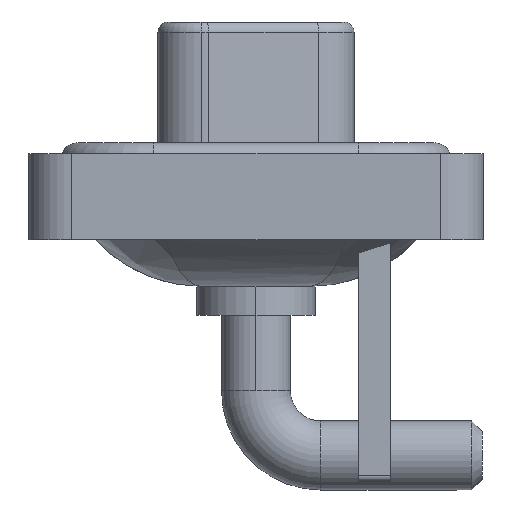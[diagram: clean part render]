
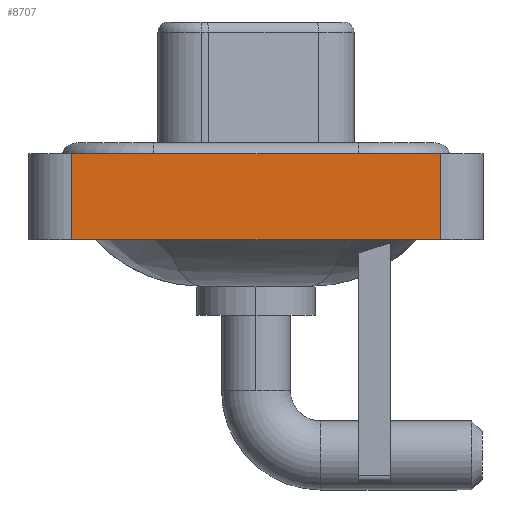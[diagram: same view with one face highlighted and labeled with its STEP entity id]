
A CAD part, left-side view. The second image highlights one B-rep face of the part: STEP entity #8707.
In plain terms, the highlighted planar face has unit normal (-1, 0, 0).
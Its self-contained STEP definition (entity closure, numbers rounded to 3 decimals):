
#892 = ORIENTED_EDGE ( 'NONE', *, *, #13719, .F. ) ;
#903 = DIRECTION ( 'NONE',  ( 0., 0., 1. ) ) ;
#2078 = LINE ( 'NONE', #10963, #12333 ) ;
#3407 = CARTESIAN_POINT ( 'NONE',  ( -7.25, 8.55, -3.6 ) ) ;
#3784 = ORIENTED_EDGE ( 'NONE', *, *, #5204, .T. ) ;
#4314 = DIRECTION ( 'NONE',  ( 0., 0., 1. ) ) ;
#5204 = EDGE_CURVE ( 'NONE', #14018, #8921, #15393, .T. ) ;
#5382 = AXIS2_PLACEMENT_3D ( 'NONE', #10099, #7242, #4314 ) ;
#5666 = VERTEX_POINT ( 'NONE', #15191 ) ;
#6091 = ORIENTED_EDGE ( 'NONE', *, *, #15179, .T. ) ;
#6730 = LINE ( 'NONE', #12501, #16020 ) ;
#6797 = DIRECTION ( 'NONE',  ( 0., -1., 0. ) ) ;
#7242 = DIRECTION ( 'NONE',  ( -1., 0., 0. ) ) ;
#7818 = DIRECTION ( 'NONE',  ( 0., -1., 0. ) ) ;
#8166 = CARTESIAN_POINT ( 'NONE',  ( -7.25, -8.55, -3.6 ) ) ;
#8707 = ADVANCED_FACE ( 'NONE', ( #10189 ), #17540, .T. ) ;
#8921 = VERTEX_POINT ( 'NONE', #8166 ) ;
#8945 = CARTESIAN_POINT ( 'NONE',  ( -7.25, 8.55, 0.4 ) ) ;
#9672 = LINE ( 'NONE', #18436, #15442 ) ;
#10099 = CARTESIAN_POINT ( 'NONE',  ( -7.25, -8.55, -3.6 ) ) ;
#10189 = FACE_OUTER_BOUND ( 'NONE', #15875, .T. ) ;
#10287 = VECTOR ( 'NONE', #6797, 1000. ) ;
#10522 = VERTEX_POINT ( 'NONE', #8945 ) ;
#10963 = CARTESIAN_POINT ( 'NONE',  ( -7.25, -8.55, 0.4 ) ) ;
#11655 = ORIENTED_EDGE ( 'NONE', *, *, #12708, .F. ) ;
#12333 = VECTOR ( 'NONE', #7818, 1000. ) ;
#12501 = CARTESIAN_POINT ( 'NONE',  ( -7.25, -8.55, -3.6 ) ) ;
#12708 = EDGE_CURVE ( 'NONE', #10522, #5666, #2078, .T. ) ;
#13719 = EDGE_CURVE ( 'NONE', #14018, #10522, #9672, .T. ) ;
#13731 = DIRECTION ( 'NONE',  ( 0., 0., 1. ) ) ;
#14018 = VERTEX_POINT ( 'NONE', #3407 ) ;
#15179 = EDGE_CURVE ( 'NONE', #8921, #5666, #6730, .T. ) ;
#15191 = CARTESIAN_POINT ( 'NONE',  ( -7.25, -8.55, 0.4 ) ) ;
#15393 = LINE ( 'NONE', #17009, #10287 ) ;
#15442 = VECTOR ( 'NONE', #903, 1000. ) ;
#15875 = EDGE_LOOP ( 'NONE', ( #6091, #11655, #892, #3784 ) ) ;
#16020 = VECTOR ( 'NONE', #13731, 1000. ) ;
#17009 = CARTESIAN_POINT ( 'NONE',  ( -7.25, -8.55, -3.6 ) ) ;
#17540 = PLANE ( 'NONE',  #5382 ) ;
#18436 = CARTESIAN_POINT ( 'NONE',  ( -7.25, 8.55, -3.6 ) ) ;
